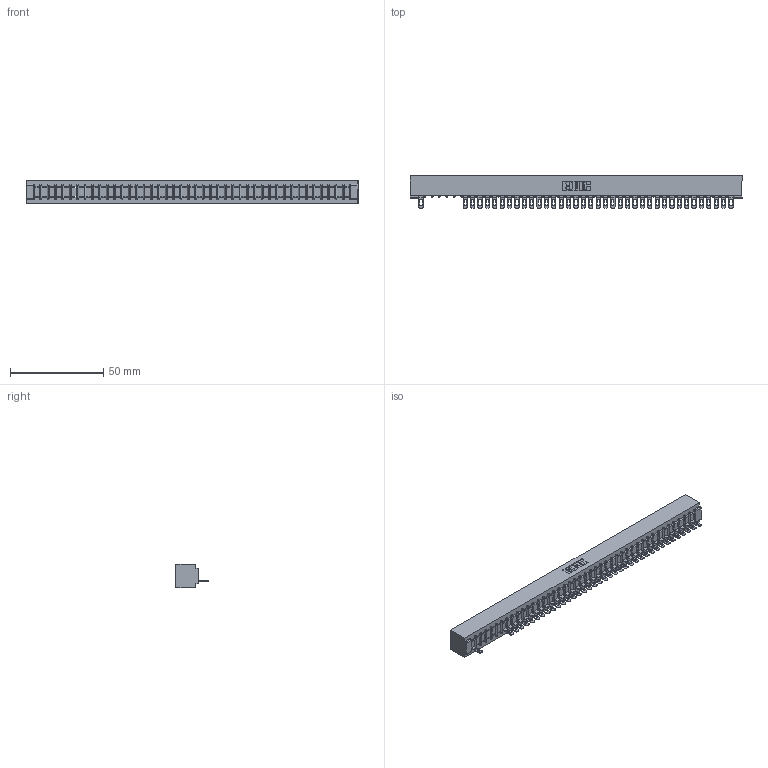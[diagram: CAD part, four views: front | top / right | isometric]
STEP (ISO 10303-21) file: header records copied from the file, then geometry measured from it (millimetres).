
FILE_DESCRIPTION (( 'STEP AP203' ), '1' );
FILE_NAME ('357-043-501-101.STEP', '2018-08-11T10:06:52', ( '' ), ( '' ), 'SwSTEP 2.0', 'SolidWorks 2016', '' );
FILE_SCHEMA (( 'CONFIG_CONTROL_DESIGN' ));
Length unit declared in the file: inch
Products named in the file (3): 307 Part_No Mounting Lugs; 307-290-002_501; 357-043-501-101
Assembly tree (39 placements, depth 2):
  357-043-501-101
    307 Part_No Mounting Lugs
    307-290-002_501  x38
Bounding box: 178.26 x 17.42 x 12.7 mm (x, y, z)
Volume: 19529.4 mm3; surface area: 24256.8 mm2
Topology: 39 solids, 39 shells, 3142 faces, 9663 edges, 6322 vertices
Faces by surface type: plane 1798, cylinder 1256, sphere 88
Entity records: 37096 total; most frequent: CARTESIAN_POINT 6279, ORIENTED_EDGE 6274, DIRECTION 6097, EDGE_CURVE 3137, LINE 2401, VECTOR 2401, VERTEX_POINT 2030, AXIS2_PLACEMENT_3D 1848
